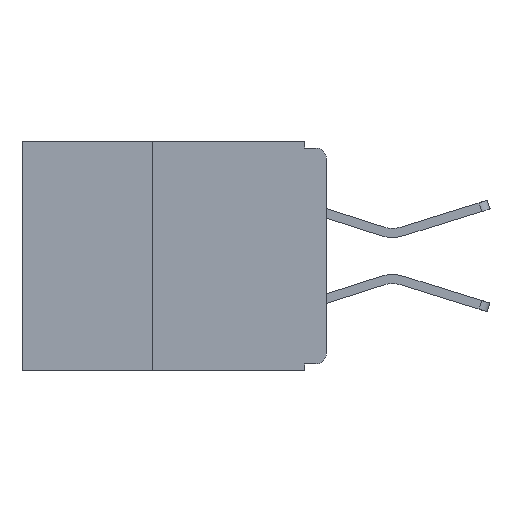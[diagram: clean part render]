
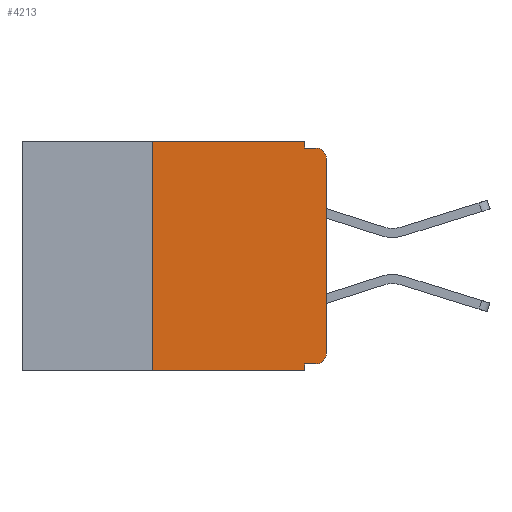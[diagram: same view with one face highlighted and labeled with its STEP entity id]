
A CAD part, left-side view. The second image highlights one B-rep face of the part: STEP entity #4213.
In plain terms, the highlighted planar face has unit normal (-1, 0, 0).
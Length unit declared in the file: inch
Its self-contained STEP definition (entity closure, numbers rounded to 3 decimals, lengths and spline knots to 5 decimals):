
#69 = ORIENTED_EDGE ( 'NONE', *, *, #16037, .F. ) ;
#261 = CARTESIAN_POINT ( 'NONE',  ( 0., 0., -0.305 ) ) ;
#403 = LINE ( 'NONE', #21868, #19232 ) ;
#704 = DIRECTION ( 'NONE',  ( 0., 0., -1. ) ) ;
#744 = CARTESIAN_POINT ( 'NONE',  ( 0., 0.031, -0.33 ) ) ;
#1534 = DIRECTION ( 'NONE',  ( 0., 0., 1. ) ) ;
#1535 = LINE ( 'NONE', #19004, #19661 ) ;
#1611 = ORIENTED_EDGE ( 'NONE', *, *, #5248, .F. ) ;
#1714 = CIRCLE ( 'NONE', #7127, 0.015 ) ;
#1728 = VERTEX_POINT ( 'NONE', #18794 ) ;
#1842 = VERTEX_POINT ( 'NONE', #18770 ) ;
#3978 = VECTOR ( 'NONE', #9791, 39.37008 ) ;
#4034 = CARTESIAN_POINT ( 'NONE',  ( 0., 0.015, -0.32 ) ) ;
#4213 = ADVANCED_FACE ( 'NONE', ( #10364 ), #10680, .F. ) ;
#4304 = CARTESIAN_POINT ( 'NONE',  ( 0., 0., -0.01 ) ) ;
#4373 = VECTOR ( 'NONE', #704, 39.37008 ) ;
#4968 = ORIENTED_EDGE ( 'NONE', *, *, #22880, .T. ) ;
#5248 = EDGE_CURVE ( 'NONE', #18583, #8986, #18077, .T. ) ;
#5852 = ORIENTED_EDGE ( 'NONE', *, *, #8770, .T. ) ;
#6014 = DIRECTION ( 'NONE',  ( 0., 1., 0. ) ) ;
#6995 = DIRECTION ( 'NONE',  ( -1., 0., 0. ) ) ;
#7127 = AXIS2_PLACEMENT_3D ( 'NONE', #17639, #6995, #19385 ) ;
#7302 = VECTOR ( 'NONE', #8289, 39.37008 ) ;
#7769 = DIRECTION ( 'NONE',  ( -1., 0., 0. ) ) ;
#7802 = LINE ( 'NONE', #8988, #21870 ) ;
#7832 = ORIENTED_EDGE ( 'NONE', *, *, #17221, .T. ) ;
#8289 = DIRECTION ( 'NONE',  ( 0., 0., -1. ) ) ;
#8770 = EDGE_CURVE ( 'NONE', #13495, #18251, #11957, .T. ) ;
#8889 = LINE ( 'NONE', #4304, #3978 ) ;
#8986 = VERTEX_POINT ( 'NONE', #15309 ) ;
#8988 = CARTESIAN_POINT ( 'NONE',  ( 0., 0.437, -0.33 ) ) ;
#9133 = VERTEX_POINT ( 'NONE', #19226 ) ;
#9769 = ORIENTED_EDGE ( 'NONE', *, *, #11154, .T. ) ;
#9791 = DIRECTION ( 'NONE',  ( 0., -1., 0. ) ) ;
#9956 = EDGE_LOOP ( 'NONE', ( #4968, #9769, #15072, #19743, #1611, #11475, #7832, #69, #19472, #5852 ) ) ;
#10113 = DIRECTION ( 'NONE',  ( 0., 0., -1. ) ) ;
#10134 = DIRECTION ( 'NONE',  ( 1., 0., 0. ) ) ;
#10364 = FACE_OUTER_BOUND ( 'NONE', #9956, .T. ) ;
#10553 = CARTESIAN_POINT ( 'NONE',  ( 0., 0.437, 0. ) ) ;
#10644 = DIRECTION ( 'NONE',  ( 0., -1., 0. ) ) ;
#10680 = PLANE ( 'NONE',  #10888 ) ;
#10798 = CARTESIAN_POINT ( 'NONE',  ( 0., 0., 0. ) ) ;
#10888 = AXIS2_PLACEMENT_3D ( 'NONE', #10553, #10134, #10113 ) ;
#10930 = CARTESIAN_POINT ( 'NONE',  ( 0., 0.25, -0.33 ) ) ;
#11154 = EDGE_CURVE ( 'NONE', #9133, #19875, #1714, .T. ) ;
#11475 = ORIENTED_EDGE ( 'NONE', *, *, #18403, .F. ) ;
#11857 = CARTESIAN_POINT ( 'NONE',  ( 0., 0.031, 0. ) ) ;
#11957 = CIRCLE ( 'NONE', #22447, 0.015 ) ;
#12843 = CARTESIAN_POINT ( 'NONE',  ( 0., 0.437, 0. ) ) ;
#13357 = LINE ( 'NONE', #10798, #22116 ) ;
#13372 = VECTOR ( 'NONE', #10644, 39.37008 ) ;
#13495 = VERTEX_POINT ( 'NONE', #4034 ) ;
#13535 = EDGE_CURVE ( 'NONE', #13495, #1842, #403, .T. ) ;
#13797 = CARTESIAN_POINT ( 'NONE',  ( 0., 0.015, -0.01 ) ) ;
#15072 = ORIENTED_EDGE ( 'NONE', *, *, #18267, .F. ) ;
#15309 = CARTESIAN_POINT ( 'NONE',  ( 0., 0.031, 0. ) ) ;
#15926 = CARTESIAN_POINT ( 'NONE',  ( 0., 0.25, 0. ) ) ;
#16037 = EDGE_CURVE ( 'NONE', #1842, #19889, #21381, .T. ) ;
#16417 = VERTEX_POINT ( 'NONE', #10930 ) ;
#17221 = EDGE_CURVE ( 'NONE', #16417, #19889, #7802, .T. ) ;
#17639 = CARTESIAN_POINT ( 'NONE',  ( 0., 0.015, -0.025 ) ) ;
#18077 = LINE ( 'NONE', #12843, #13372 ) ;
#18104 = LINE ( 'NONE', #11857, #4373 ) ;
#18251 = VERTEX_POINT ( 'NONE', #261 ) ;
#18267 = EDGE_CURVE ( 'NONE', #1728, #19875, #8889, .T. ) ;
#18402 = CARTESIAN_POINT ( 'NONE',  ( 0., 0.015, -0.305 ) ) ;
#18403 = EDGE_CURVE ( 'NONE', #16417, #18583, #1535, .T. ) ;
#18583 = VERTEX_POINT ( 'NONE', #15926 ) ;
#18770 = CARTESIAN_POINT ( 'NONE',  ( 0., 0.031, -0.32 ) ) ;
#18794 = CARTESIAN_POINT ( 'NONE',  ( 0., 0.031, -0.01 ) ) ;
#19004 = CARTESIAN_POINT ( 'NONE',  ( 0., 0.25, -0.33 ) ) ;
#19023 = CARTESIAN_POINT ( 'NONE',  ( 0., 0.031, -0.33 ) ) ;
#19226 = CARTESIAN_POINT ( 'NONE',  ( 0., 0., -0.025 ) ) ;
#19232 = VECTOR ( 'NONE', #6014, 39.37008 ) ;
#19385 = DIRECTION ( 'NONE',  ( 0., 0., -1. ) ) ;
#19472 = ORIENTED_EDGE ( 'NONE', *, *, #13535, .F. ) ;
#19661 = VECTOR ( 'NONE', #20739, 39.37008 ) ;
#19743 = ORIENTED_EDGE ( 'NONE', *, *, #21877, .F. ) ;
#19875 = VERTEX_POINT ( 'NONE', #13797 ) ;
#19889 = VERTEX_POINT ( 'NONE', #19023 ) ;
#20143 = DIRECTION ( 'NONE',  ( 0., 0., -1. ) ) ;
#20739 = DIRECTION ( 'NONE',  ( 0., 0., 1. ) ) ;
#21309 = DIRECTION ( 'NONE',  ( 0., -1., 0. ) ) ;
#21381 = LINE ( 'NONE', #744, #7302 ) ;
#21868 = CARTESIAN_POINT ( 'NONE',  ( 0., 0., -0.32 ) ) ;
#21870 = VECTOR ( 'NONE', #21309, 39.37008 ) ;
#21877 = EDGE_CURVE ( 'NONE', #8986, #1728, #18104, .T. ) ;
#22116 = VECTOR ( 'NONE', #1534, 39.37008 ) ;
#22447 = AXIS2_PLACEMENT_3D ( 'NONE', #18402, #7769, #20143 ) ;
#22880 = EDGE_CURVE ( 'NONE', #18251, #9133, #13357, .T. ) ;
